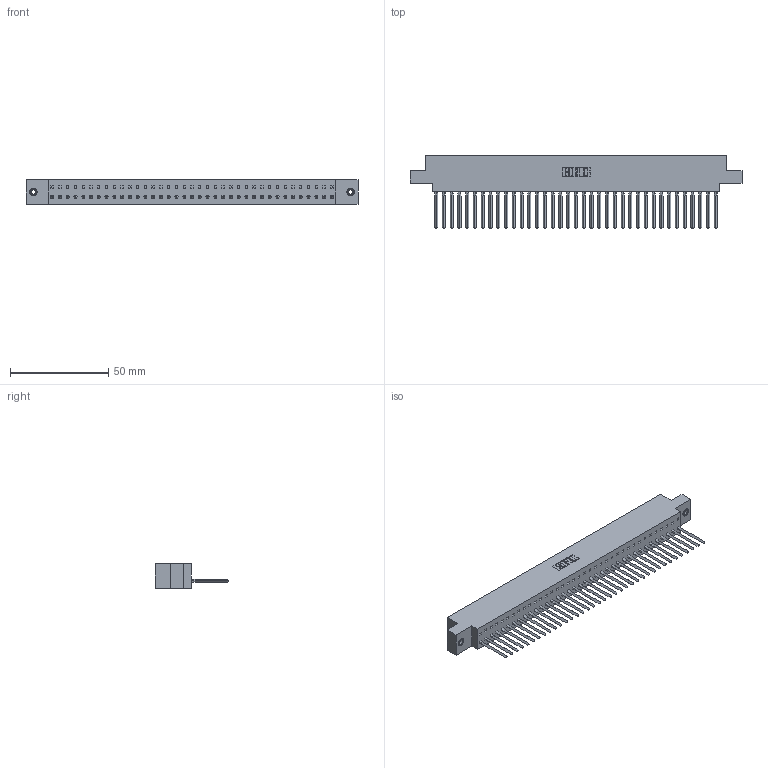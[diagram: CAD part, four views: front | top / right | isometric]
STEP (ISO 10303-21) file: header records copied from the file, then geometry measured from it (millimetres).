
FILE_DESCRIPTION (( 'STEP AP203' ), '1' );
FILE_NAME ('317-037-541-608.STEP', '2020-02-27T23:16:01', ( '' ), ( '' ), 'SwSTEP 2.0', 'SolidWorks 2016', '' );
FILE_SCHEMA (( 'CONFIG_CONTROL_DESIGN' ));
Length unit declared in the file: inch
Products named in the file (4): 317-290-002_541; 345-250-001_345-250-003-102; 317 Part_.156 Dia - TI; 317-037-541-608
Assembly tree (40 placements, depth 2):
  317-037-541-608
    317 Part_.156 Dia - TI
    317-290-002_541  x37
    345-250-001_345-250-003-102  x2
Bounding box: 169.32 x 37.34 x 12.7 mm (x, y, z)
Volume: 27297.2 mm3; surface area: 38427.6 mm2
Topology: 40 solids, 40 shells, 5786 faces, 16469 edges, 10700 vertices
Faces by surface type: plane 4678, cylinder 944, bspline 148, cone 12, torus 4
Entity records: 55731 total; most frequent: CARTESIAN_POINT 10515, ORIENTED_EDGE 9798, DIRECTION 8087, EDGE_CURVE 4899, LINE 4515, VECTOR 4515, VERTEX_POINT 3254, AXIS2_PLACEMENT_3D 1786
